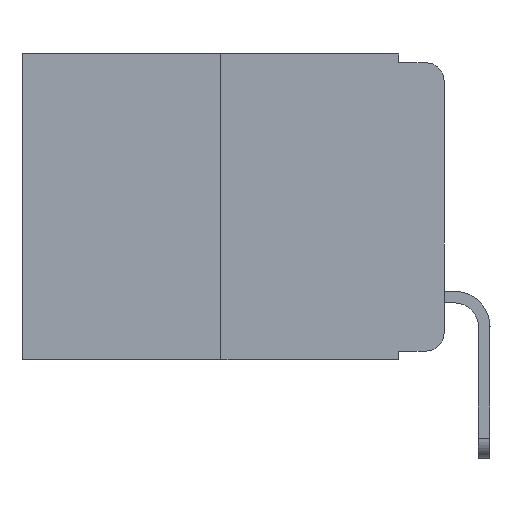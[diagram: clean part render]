
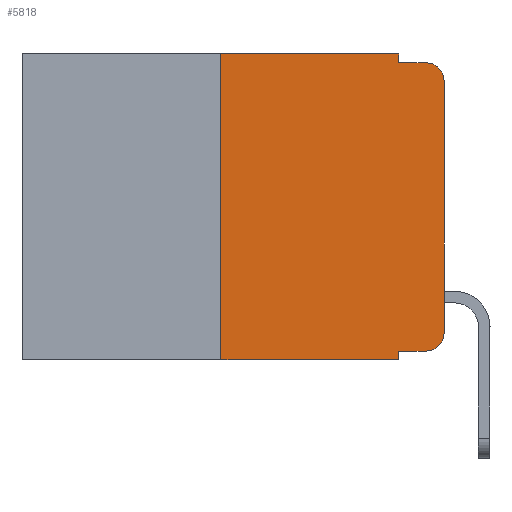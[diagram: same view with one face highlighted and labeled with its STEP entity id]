
A CAD part, left-side view. The second image highlights one B-rep face of the part: STEP entity #5818.
In plain terms, the highlighted planar face has unit normal (-1, 0, 0).
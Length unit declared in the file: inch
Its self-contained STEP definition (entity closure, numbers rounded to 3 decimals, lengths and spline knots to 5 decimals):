
#123 = VECTOR ( 'NONE', #4111, 39.37008 ) ;
#199 = DIRECTION ( 'NONE',  ( 0., 0., -1. ) ) ;
#475 = EDGE_LOOP ( 'NONE', ( #18534, #13788, #4962, #21710, #14454, #6783, #19995, #16908, #16960, #4894 ) ) ;
#715 = VECTOR ( 'NONE', #19563, 39.37008 ) ;
#1125 = CARTESIAN_POINT ( 'NONE',  ( 0., 0.051, -0.01 ) ) ;
#1237 = VERTEX_POINT ( 'NONE', #11303 ) ;
#1426 = CARTESIAN_POINT ( 'NONE',  ( 0., 0.051, -0.01 ) ) ;
#1539 = VERTEX_POINT ( 'NONE', #8987 ) ;
#1842 = EDGE_CURVE ( 'NONE', #14255, #19773, #13189, .T. ) ;
#1986 = DIRECTION ( 'NONE',  ( 0., 0., -1. ) ) ;
#2117 = CARTESIAN_POINT ( 'NONE',  ( 0., 0.051, 0. ) ) ;
#2458 = EDGE_CURVE ( 'NONE', #14250, #1237, #21752, .T. ) ;
#2577 = EDGE_CURVE ( 'NONE', #1539, #19773, #13549, .T. ) ;
#2705 = DIRECTION ( 'NONE',  ( 0., 0., -1. ) ) ;
#3441 = DIRECTION ( 'NONE',  ( 1., 0., 0. ) ) ;
#3695 = EDGE_CURVE ( 'NONE', #4250, #8378, #11882, .T. ) ;
#4111 = DIRECTION ( 'NONE',  ( 0., -1., 0. ) ) ;
#4250 = VERTEX_POINT ( 'NONE', #7787 ) ;
#4363 = CARTESIAN_POINT ( 'NONE',  ( 0., 0.051, -0.333 ) ) ;
#4493 = EDGE_CURVE ( 'NONE', #11742, #8378, #11289, .T. ) ;
#4894 = ORIENTED_EDGE ( 'NONE', *, *, #5344, .T. ) ;
#4962 = ORIENTED_EDGE ( 'NONE', *, *, #1842, .F. ) ;
#5047 = DIRECTION ( 'NONE',  ( 0., -1., 0. ) ) ;
#5344 = EDGE_CURVE ( 'NONE', #22352, #6662, #16369, .T. ) ;
#5818 = ADVANCED_FACE ( 'NONE', ( #9677 ), #22878, .F. ) ;
#5907 = LINE ( 'NONE', #23069, #9953 ) ;
#6254 = DIRECTION ( 'NONE',  ( 0., -1., 0. ) ) ;
#6662 = VERTEX_POINT ( 'NONE', #7222 ) ;
#6783 = ORIENTED_EDGE ( 'NONE', *, *, #21994, .F. ) ;
#6863 = CARTESIAN_POINT ( 'NONE',  ( 0., 0.02, -0.333 ) ) ;
#7102 = VECTOR ( 'NONE', #14606, 39.37008 ) ;
#7222 = CARTESIAN_POINT ( 'NONE',  ( 0., 0., -0.313 ) ) ;
#7787 = CARTESIAN_POINT ( 'NONE',  ( 0., 0.051, -0.333 ) ) ;
#8173 = LINE ( 'NONE', #4363, #14547 ) ;
#8236 = LINE ( 'NONE', #23499, #715 ) ;
#8378 = VERTEX_POINT ( 'NONE', #24273 ) ;
#8987 = CARTESIAN_POINT ( 'NONE',  ( 0., 0., -0.03 ) ) ;
#9677 = FACE_OUTER_BOUND ( 'NONE', #475, .T. ) ;
#9709 = VECTOR ( 'NONE', #5047, 39.37008 ) ;
#9953 = VECTOR ( 'NONE', #1986, 39.37008 ) ;
#11190 = DIRECTION ( 'NONE',  ( 0., 0., -1. ) ) ;
#11289 = LINE ( 'NONE', #21063, #21019 ) ;
#11303 = CARTESIAN_POINT ( 'NONE',  ( 0., 0.051, 0. ) ) ;
#11491 = CARTESIAN_POINT ( 'NONE',  ( 0., 0.25, -0.343 ) ) ;
#11607 = VECTOR ( 'NONE', #199, 39.37008 ) ;
#11742 = VERTEX_POINT ( 'NONE', #11491 ) ;
#11882 = LINE ( 'NONE', #2117, #11607 ) ;
#12593 = CARTESIAN_POINT ( 'NONE',  ( 0., 0.02, -0.03 ) ) ;
#12732 = CARTESIAN_POINT ( 'NONE',  ( 0., 0.25, 0. ) ) ;
#13019 = EDGE_CURVE ( 'NONE', #1237, #14255, #5907, .T. ) ;
#13189 = LINE ( 'NONE', #1125, #9709 ) ;
#13516 = CARTESIAN_POINT ( 'NONE',  ( 0., 0.02, -0.01 ) ) ;
#13549 = CIRCLE ( 'NONE', #15157, 0.02 ) ;
#13781 = CARTESIAN_POINT ( 'NONE',  ( 0., 0.02, -0.313 ) ) ;
#13788 = ORIENTED_EDGE ( 'NONE', *, *, #2577, .T. ) ;
#14250 = VERTEX_POINT ( 'NONE', #12732 ) ;
#14255 = VERTEX_POINT ( 'NONE', #1426 ) ;
#14454 = ORIENTED_EDGE ( 'NONE', *, *, #2458, .F. ) ;
#14547 = VECTOR ( 'NONE', #6254, 39.37008 ) ;
#14606 = DIRECTION ( 'NONE',  ( 0., 0., 1. ) ) ;
#15151 = EDGE_CURVE ( 'NONE', #6662, #1539, #16497, .T. ) ;
#15157 = AXIS2_PLACEMENT_3D ( 'NONE', #12593, #22366, #2705 ) ;
#16369 = CIRCLE ( 'NONE', #22846, 0.02 ) ;
#16497 = LINE ( 'NONE', #18645, #7102 ) ;
#16908 = ORIENTED_EDGE ( 'NONE', *, *, #3695, .F. ) ;
#16960 = ORIENTED_EDGE ( 'NONE', *, *, #22226, .T. ) ;
#18534 = ORIENTED_EDGE ( 'NONE', *, *, #15151, .T. ) ;
#18645 = CARTESIAN_POINT ( 'NONE',  ( 0., 0., 0. ) ) ;
#19038 = DIRECTION ( 'NONE',  ( 0., -1., 0. ) ) ;
#19106 = DIRECTION ( 'NONE',  ( 0., 0., -1. ) ) ;
#19563 = DIRECTION ( 'NONE',  ( 0., 0., 1. ) ) ;
#19773 = VERTEX_POINT ( 'NONE', #13516 ) ;
#19995 = ORIENTED_EDGE ( 'NONE', *, *, #4493, .T. ) ;
#20828 = CARTESIAN_POINT ( 'NONE',  ( 0., 0.473, 0. ) ) ;
#21019 = VECTOR ( 'NONE', #19038, 39.37008 ) ;
#21063 = CARTESIAN_POINT ( 'NONE',  ( 0., 0.473, -0.343 ) ) ;
#21498 = CARTESIAN_POINT ( 'NONE',  ( 0., 0.473, 0. ) ) ;
#21710 = ORIENTED_EDGE ( 'NONE', *, *, #13019, .F. ) ;
#21752 = LINE ( 'NONE', #21498, #123 ) ;
#21923 = AXIS2_PLACEMENT_3D ( 'NONE', #20828, #3441, #11190 ) ;
#21994 = EDGE_CURVE ( 'NONE', #11742, #14250, #8236, .T. ) ;
#22226 = EDGE_CURVE ( 'NONE', #4250, #22352, #8173, .T. ) ;
#22352 = VERTEX_POINT ( 'NONE', #6863 ) ;
#22366 = DIRECTION ( 'NONE',  ( -1., 0., 0. ) ) ;
#22846 = AXIS2_PLACEMENT_3D ( 'NONE', #13781, #23307, #19106 ) ;
#22878 = PLANE ( 'NONE',  #21923 ) ;
#23069 = CARTESIAN_POINT ( 'NONE',  ( 0., 0.051, 0. ) ) ;
#23307 = DIRECTION ( 'NONE',  ( -1., 0., 0. ) ) ;
#23499 = CARTESIAN_POINT ( 'NONE',  ( 0., 0.25, 0. ) ) ;
#24273 = CARTESIAN_POINT ( 'NONE',  ( 0., 0.051, -0.343 ) ) ;
